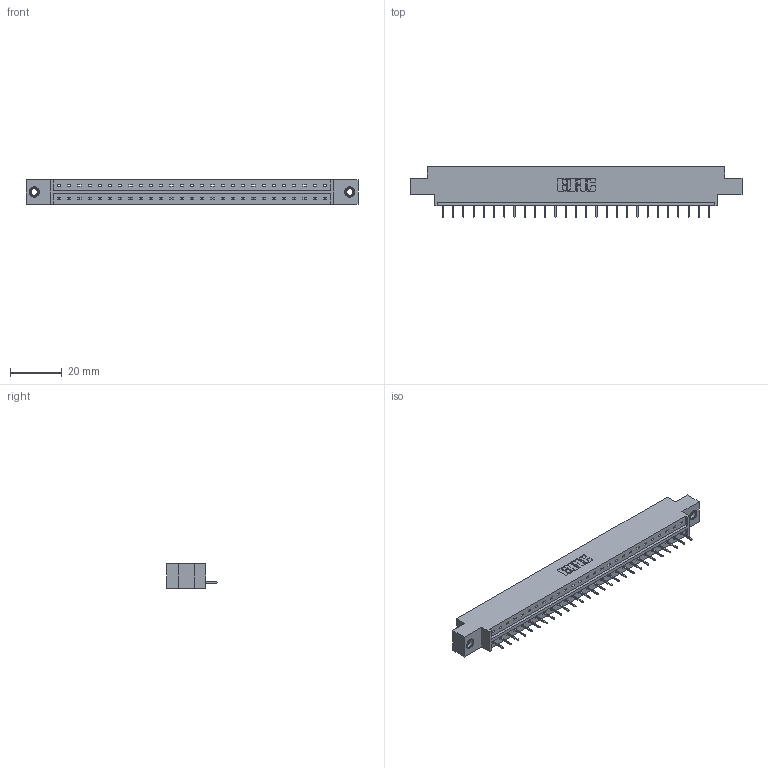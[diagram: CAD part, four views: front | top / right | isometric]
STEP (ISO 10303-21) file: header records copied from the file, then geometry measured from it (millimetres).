
FILE_DESCRIPTION (( 'STEP AP203' ), '1' );
FILE_NAME ('333-027-524-607.STEP', '2018-08-02T13:57:10', ( '' ), ( '' ), 'SwSTEP 2.0', 'SolidWorks 2016', '' );
FILE_SCHEMA (( 'CONFIG_CONTROL_DESIGN' ));
Length unit declared in the file: inch
Products named in the file (4): 333 Part_Offset - .156 Dia - TI; 345-292-001_345-293-124; 345-250-001_345-250-005-103; 333-027-524-607
Assembly tree (30 placements, depth 2):
  333-027-524-607
    333 Part_Offset - .156 Dia - TI
    345-292-001_345-293-124  x27
    345-250-001_345-250-005-103  x2
Bounding box: 128.52 x 19.69 x 9.4 mm (x, y, z)
Volume: 12456.2 mm3; surface area: 13248.2 mm2
Topology: 30 solids, 30 shells, 1852 faces, 5319 edges, 3430 vertices
Faces by surface type: plane 1402, cylinder 434, cone 12, torus 4
Entity records: 19838 total; most frequent: CARTESIAN_POINT 3406, ORIENTED_EDGE 3362, DIRECTION 2937, EDGE_CURVE 1681, VECTOR 1537, LINE 1537, VERTEX_POINT 1112, AXIS2_PLACEMENT_3D 700
